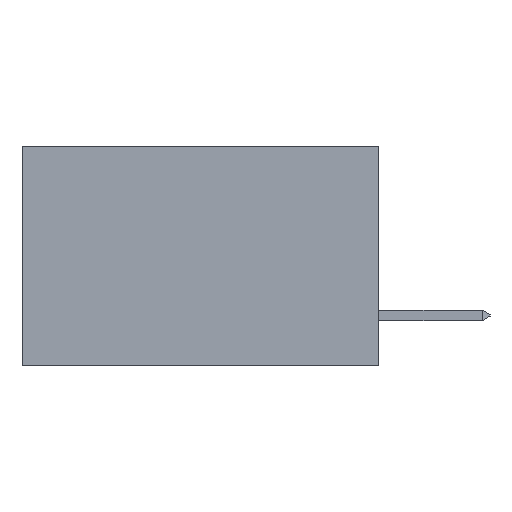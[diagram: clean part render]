
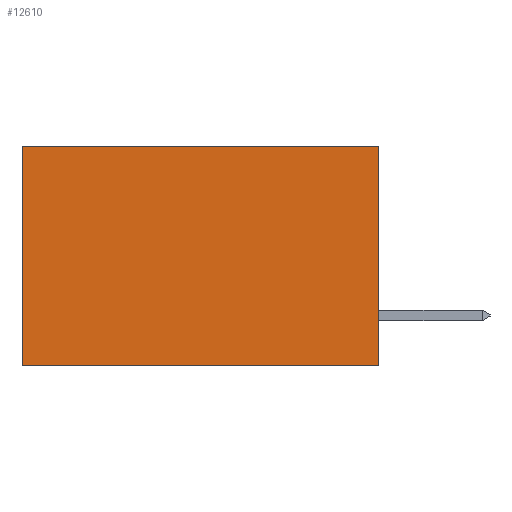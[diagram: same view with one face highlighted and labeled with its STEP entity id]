
A CAD part, left-side view. The second image highlights one B-rep face of the part: STEP entity #12610.
In plain terms, the highlighted planar face has unit normal (-1, 0, 0).
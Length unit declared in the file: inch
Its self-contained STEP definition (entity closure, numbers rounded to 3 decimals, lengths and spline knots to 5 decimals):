
#226 = DIRECTION ( 'NONE',  ( 0., 0., -1. ) ) ;
#256 = DIRECTION ( 'NONE',  ( 1., 0., 0. ) ) ;
#845 = EDGE_CURVE ( 'NONE', #1997, #1141, #7633, .T. ) ;
#1141 = VERTEX_POINT ( 'NONE', #13444 ) ;
#1540 = VERTEX_POINT ( 'NONE', #15046 ) ;
#1997 = VERTEX_POINT ( 'NONE', #10987 ) ;
#3418 = VECTOR ( 'NONE', #10716, 39.37008 ) ;
#3768 = VECTOR ( 'NONE', #6774, 39.37008 ) ;
#4428 = VECTOR ( 'NONE', #13773, 39.37008 ) ;
#4459 = CARTESIAN_POINT ( 'NONE',  ( 0.2615, 0., 0. ) ) ;
#5134 = ORIENTED_EDGE ( 'NONE', *, *, #8267, .F. ) ;
#6520 = ORIENTED_EDGE ( 'NONE', *, *, #15068, .T. ) ;
#6721 = PLANE ( 'NONE',  #10879 ) ;
#6774 = DIRECTION ( 'NONE',  ( 0., 1., 0. ) ) ;
#7633 = LINE ( 'NONE', #4459, #3768 ) ;
#7666 = VECTOR ( 'NONE', #226, 39.37008 ) ;
#8267 = EDGE_CURVE ( 'NONE', #1540, #13846, #11252, .T. ) ;
#8301 = EDGE_LOOP ( 'NONE', ( #6520, #5134, #14172, #15489 ) ) ;
#8559 = EDGE_CURVE ( 'NONE', #1997, #1540, #13565, .T. ) ;
#9270 = CARTESIAN_POINT ( 'NONE',  ( 0.2615, 0.6, -0.37 ) ) ;
#9295 = DIRECTION ( 'NONE',  ( 0., 0., -1. ) ) ;
#9540 = FACE_OUTER_BOUND ( 'NONE', #8301, .T. ) ;
#10522 = CARTESIAN_POINT ( 'NONE',  ( 0.2615, 0.6, -0.37 ) ) ;
#10716 = DIRECTION ( 'NONE',  ( 0., 0., -1. ) ) ;
#10879 = AXIS2_PLACEMENT_3D ( 'NONE', #15449, #256, #9295 ) ;
#10987 = CARTESIAN_POINT ( 'NONE',  ( 0.2615, 0., 0. ) ) ;
#11017 = CARTESIAN_POINT ( 'NONE',  ( 0.2615, 0., -0.37 ) ) ;
#11252 = LINE ( 'NONE', #13849, #4428 ) ;
#12610 = ADVANCED_FACE ( 'NONE', ( #9540 ), #6721, .F. ) ;
#13444 = CARTESIAN_POINT ( 'NONE',  ( 0.2615, 0.6, 0. ) ) ;
#13565 = LINE ( 'NONE', #11017, #3418 ) ;
#13773 = DIRECTION ( 'NONE',  ( 0., 1., 0. ) ) ;
#13846 = VERTEX_POINT ( 'NONE', #10522 ) ;
#13849 = CARTESIAN_POINT ( 'NONE',  ( 0.2615, 0., -0.37 ) ) ;
#13945 = LINE ( 'NONE', #9270, #7666 ) ;
#14172 = ORIENTED_EDGE ( 'NONE', *, *, #8559, .F. ) ;
#15046 = CARTESIAN_POINT ( 'NONE',  ( 0.2615, 0., -0.37 ) ) ;
#15068 = EDGE_CURVE ( 'NONE', #1141, #13846, #13945, .T. ) ;
#15449 = CARTESIAN_POINT ( 'NONE',  ( 0.2615, 0., -0.37 ) ) ;
#15489 = ORIENTED_EDGE ( 'NONE', *, *, #845, .T. ) ;
